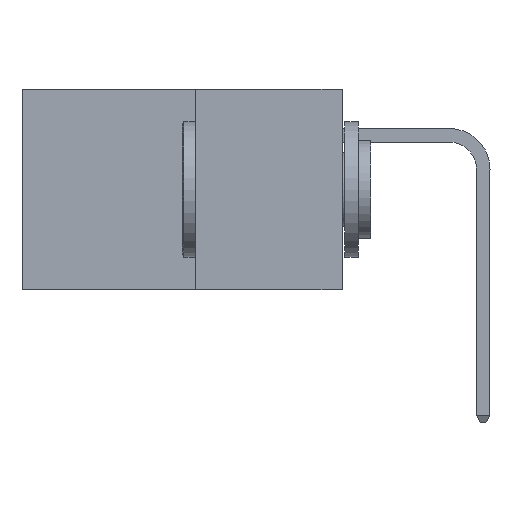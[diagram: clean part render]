
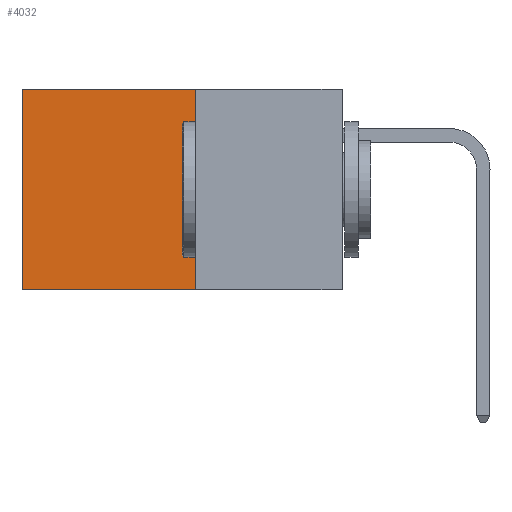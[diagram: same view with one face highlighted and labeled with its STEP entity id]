
A CAD part, left-side view. The second image highlights one B-rep face of the part: STEP entity #4032.
In plain terms, the highlighted planar face has unit normal (-1, 0, 0).
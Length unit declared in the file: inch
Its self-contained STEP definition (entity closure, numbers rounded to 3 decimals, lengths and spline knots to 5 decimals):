
#506 = VECTOR ( 'NONE', #3668, 39.37008 ) ;
#1033 = LINE ( 'NONE', #11488, #5749 ) ;
#1053 = EDGE_CURVE ( 'NONE', #11321, #1330, #11850, .T. ) ;
#1330 = VERTEX_POINT ( 'NONE', #3003 ) ;
#1372 = VECTOR ( 'NONE', #12587, 39.37008 ) ;
#1517 = DIRECTION ( 'NONE',  ( 0., 0., -1. ) ) ;
#1732 = EDGE_CURVE ( 'NONE', #11321, #9962, #1033, .T. ) ;
#1843 = EDGE_CURVE ( 'NONE', #9962, #11498, #6255, .T. ) ;
#1972 = EDGE_LOOP ( 'NONE', ( #12371, #2277, #12665, #2639 ) ) ;
#2277 = ORIENTED_EDGE ( 'NONE', *, *, #11728, .F. ) ;
#2353 = CARTESIAN_POINT ( 'NONE',  ( 0.277, 0.59, -0.37 ) ) ;
#2639 = ORIENTED_EDGE ( 'NONE', *, *, #1732, .T. ) ;
#2676 = DIRECTION ( 'NONE',  ( 0., 1., 0. ) ) ;
#3003 = CARTESIAN_POINT ( 'NONE',  ( 0.277, 0.27, -0.37 ) ) ;
#3668 = DIRECTION ( 'NONE',  ( 0., 1., 0. ) ) ;
#3706 = DIRECTION ( 'NONE',  ( 0., 0., -1. ) ) ;
#3723 = DIRECTION ( 'NONE',  ( 1., 0., 0. ) ) ;
#3808 = PLANE ( 'NONE',  #8749 ) ;
#3850 = CARTESIAN_POINT ( 'NONE',  ( 0.277, 0.27, -0.37 ) ) ;
#4032 = ADVANCED_FACE ( 'NONE', ( #11825 ), #3808, .F. ) ;
#4517 = CARTESIAN_POINT ( 'NONE',  ( 0.277, 0.27, -0.37 ) ) ;
#5357 = CARTESIAN_POINT ( 'NONE',  ( 0.277, 0.59, -0.37 ) ) ;
#5749 = VECTOR ( 'NONE', #2676, 39.37008 ) ;
#6255 = LINE ( 'NONE', #2353, #8559 ) ;
#7189 = CARTESIAN_POINT ( 'NONE',  ( 0.277, 0.27, 0. ) ) ;
#8161 = LINE ( 'NONE', #11446, #506 ) ;
#8559 = VECTOR ( 'NONE', #1517, 39.37008 ) ;
#8749 = AXIS2_PLACEMENT_3D ( 'NONE', #3850, #3723, #3706 ) ;
#9158 = CARTESIAN_POINT ( 'NONE',  ( 0.277, 0.59, 0. ) ) ;
#9962 = VERTEX_POINT ( 'NONE', #9158 ) ;
#11321 = VERTEX_POINT ( 'NONE', #7189 ) ;
#11446 = CARTESIAN_POINT ( 'NONE',  ( 0.277, 0.27, -0.37 ) ) ;
#11488 = CARTESIAN_POINT ( 'NONE',  ( 0.277, 0.27, 0. ) ) ;
#11498 = VERTEX_POINT ( 'NONE', #5357 ) ;
#11728 = EDGE_CURVE ( 'NONE', #1330, #11498, #8161, .T. ) ;
#11825 = FACE_OUTER_BOUND ( 'NONE', #1972, .T. ) ;
#11850 = LINE ( 'NONE', #4517, #1372 ) ;
#12371 = ORIENTED_EDGE ( 'NONE', *, *, #1843, .T. ) ;
#12587 = DIRECTION ( 'NONE',  ( 0., 0., -1. ) ) ;
#12665 = ORIENTED_EDGE ( 'NONE', *, *, #1053, .F. ) ;
